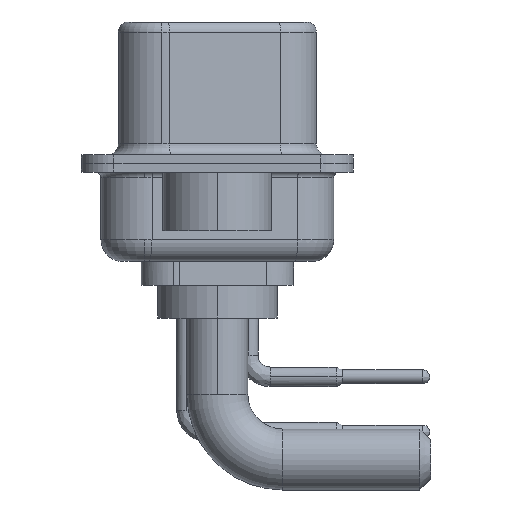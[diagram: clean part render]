
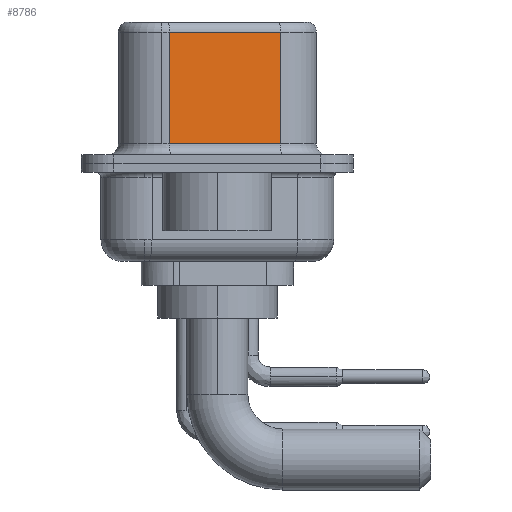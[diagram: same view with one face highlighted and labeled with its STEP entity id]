
A CAD part, left-side view. The second image highlights one B-rep face of the part: STEP entity #8786.
In plain terms, the highlighted planar face has unit normal (-0.985, -0.174, 0).
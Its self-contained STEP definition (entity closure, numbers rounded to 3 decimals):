
#183 = EDGE_LOOP ( 'NONE', ( #7958, #15031, #8488, #20505 ) ) ;
#694 = VECTOR ( 'NONE', #15882, 1000. ) ;
#1021 = EDGE_CURVE ( 'NONE', #16663, #5589, #11312, .T. ) ;
#1475 = DIRECTION ( 'NONE',  ( 0.985, 0.174, 0. ) ) ;
#1888 = LINE ( 'NONE', #14831, #19766 ) ;
#1908 = VECTOR ( 'NONE', #18293, 1000. ) ;
#5274 = CARTESIAN_POINT ( 'NONE',  ( 4.555, -2.897, 6.02 ) ) ;
#5589 = VERTEX_POINT ( 'NONE', #9954 ) ;
#5837 = CARTESIAN_POINT ( 'NONE',  ( 3.655, 2.203, 6.02 ) ) ;
#6108 = CARTESIAN_POINT ( 'NONE',  ( 3.655, 2.203, 6.52 ) ) ;
#6126 = FACE_OUTER_BOUND ( 'NONE', #183, .T. ) ;
#7958 = ORIENTED_EDGE ( 'NONE', *, *, #12660, .F. ) ;
#8412 = LINE ( 'NONE', #9907, #1908 ) ;
#8488 = ORIENTED_EDGE ( 'NONE', *, *, #1021, .T. ) ;
#8786 = ADVANCED_FACE ( 'NONE', ( #6126 ), #19065, .F. ) ;
#9517 = CARTESIAN_POINT ( 'NONE',  ( 4.555, -2.897, 6.52 ) ) ;
#9907 = CARTESIAN_POINT ( 'NONE',  ( 4.555, -2.897, 6.02 ) ) ;
#9954 = CARTESIAN_POINT ( 'NONE',  ( 3.655, 2.203, 0.9 ) ) ;
#11312 = LINE ( 'NONE', #6108, #694 ) ;
#12308 = CARTESIAN_POINT ( 'NONE',  ( 4.555, -2.897, 6.52 ) ) ;
#12660 = EDGE_CURVE ( 'NONE', #17324, #13110, #16981, .T. ) ;
#13110 = VERTEX_POINT ( 'NONE', #14303 ) ;
#14303 = CARTESIAN_POINT ( 'NONE',  ( 4.555, -2.897, 0.9 ) ) ;
#14420 = DIRECTION ( 'NONE',  ( -0.174, 0.985, 0. ) ) ;
#14831 = CARTESIAN_POINT ( 'NONE',  ( 4.555, -2.897, 0.9 ) ) ;
#15031 = ORIENTED_EDGE ( 'NONE', *, *, #15094, .T. ) ;
#15094 = EDGE_CURVE ( 'NONE', #17324, #16663, #8412, .T. ) ;
#15390 = VECTOR ( 'NONE', #18565, 1000. ) ;
#15882 = DIRECTION ( 'NONE',  ( 0., 0., -1. ) ) ;
#16663 = VERTEX_POINT ( 'NONE', #5837 ) ;
#16981 = LINE ( 'NONE', #12308, #15390 ) ;
#17324 = VERTEX_POINT ( 'NONE', #5274 ) ;
#17397 = EDGE_CURVE ( 'NONE', #5589, #13110, #1888, .T. ) ;
#18293 = DIRECTION ( 'NONE',  ( -0.174, 0.985, 0. ) ) ;
#18565 = DIRECTION ( 'NONE',  ( 0., 0., -1. ) ) ;
#19065 = PLANE ( 'NONE',  #19321 ) ;
#19321 = AXIS2_PLACEMENT_3D ( 'NONE', #9517, #1475, #14420 ) ;
#19766 = VECTOR ( 'NONE', #19793, 1000. ) ;
#19793 = DIRECTION ( 'NONE',  ( 0.174, -0.985, 0. ) ) ;
#20505 = ORIENTED_EDGE ( 'NONE', *, *, #17397, .T. ) ;
